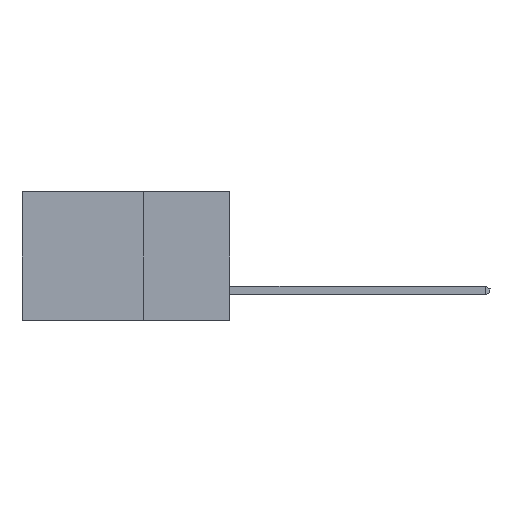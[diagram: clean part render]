
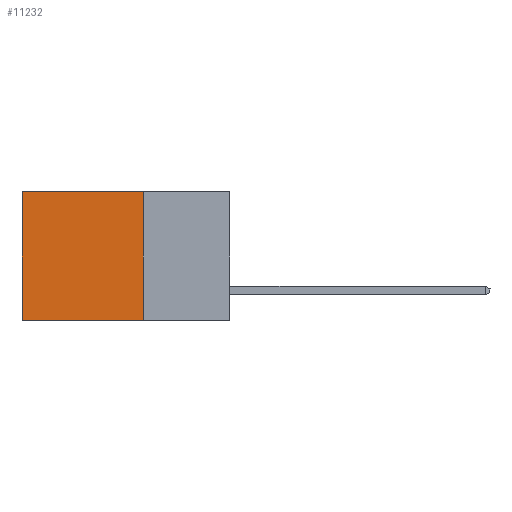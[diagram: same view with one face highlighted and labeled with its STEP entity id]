
A CAD part, left-side view. The second image highlights one B-rep face of the part: STEP entity #11232.
In plain terms, the highlighted planar face has unit normal (-1, 0, 0).
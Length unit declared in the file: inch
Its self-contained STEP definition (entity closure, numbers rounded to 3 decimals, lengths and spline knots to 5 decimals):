
#88 = LINE ( 'NONE', #11737, #9598 ) ;
#199 = DIRECTION ( 'NONE',  ( 0., 1., 0. ) ) ;
#221 = DIRECTION ( 'NONE',  ( 0., 0., -1. ) ) ;
#704 = DIRECTION ( 'NONE',  ( 0., 0., -1. ) ) ;
#1041 = LINE ( 'NONE', #12473, #8556 ) ;
#1166 = EDGE_CURVE ( 'NONE', #5690, #11440, #5392, .T. ) ;
#1561 = VECTOR ( 'NONE', #11992, 39.37008 ) ;
#1799 = ORIENTED_EDGE ( 'NONE', *, *, #5631, .F. ) ;
#2341 = CARTESIAN_POINT ( 'NONE',  ( 0.2615, 0.6, -0.37 ) ) ;
#3004 = CARTESIAN_POINT ( 'NONE',  ( 0.2615, 0.6, 0. ) ) ;
#3561 = VERTEX_POINT ( 'NONE', #3004 ) ;
#3875 = ORIENTED_EDGE ( 'NONE', *, *, #1166, .F. ) ;
#3984 = DIRECTION ( 'NONE',  ( 1., 0., 0. ) ) ;
#4280 = CARTESIAN_POINT ( 'NONE',  ( 0.2615, 0.25, -0.37 ) ) ;
#5392 = LINE ( 'NONE', #9681, #10831 ) ;
#5631 = EDGE_CURVE ( 'NONE', #10891, #5690, #88, .T. ) ;
#5690 = VERTEX_POINT ( 'NONE', #4280 ) ;
#5800 = CARTESIAN_POINT ( 'NONE',  ( 0.2615, 0.25, 0. ) ) ;
#6017 = PLANE ( 'NONE',  #13345 ) ;
#6875 = LINE ( 'NONE', #5800, #1561 ) ;
#7018 = EDGE_CURVE ( 'NONE', #10891, #3561, #6875, .T. ) ;
#7914 = EDGE_CURVE ( 'NONE', #3561, #11440, #1041, .T. ) ;
#7997 = FACE_OUTER_BOUND ( 'NONE', #12380, .T. ) ;
#8160 = ORIENTED_EDGE ( 'NONE', *, *, #7914, .T. ) ;
#8207 = DIRECTION ( 'NONE',  ( 0., 0., -1. ) ) ;
#8556 = VECTOR ( 'NONE', #8207, 39.37008 ) ;
#9427 = CARTESIAN_POINT ( 'NONE',  ( 0.2615, 0.25, 0. ) ) ;
#9598 = VECTOR ( 'NONE', #221, 39.37008 ) ;
#9681 = CARTESIAN_POINT ( 'NONE',  ( 0.2615, 0.25, -0.37 ) ) ;
#10831 = VECTOR ( 'NONE', #199, 39.37008 ) ;
#10891 = VERTEX_POINT ( 'NONE', #9427 ) ;
#10917 = ORIENTED_EDGE ( 'NONE', *, *, #7018, .T. ) ;
#11034 = CARTESIAN_POINT ( 'NONE',  ( 0.2615, 0.25, -0.37 ) ) ;
#11232 = ADVANCED_FACE ( 'NONE', ( #7997 ), #6017, .F. ) ;
#11440 = VERTEX_POINT ( 'NONE', #2341 ) ;
#11737 = CARTESIAN_POINT ( 'NONE',  ( 0.2615, 0.25, -0.37 ) ) ;
#11992 = DIRECTION ( 'NONE',  ( 0., 1., 0. ) ) ;
#12380 = EDGE_LOOP ( 'NONE', ( #8160, #3875, #1799, #10917 ) ) ;
#12473 = CARTESIAN_POINT ( 'NONE',  ( 0.2615, 0.6, -0.37 ) ) ;
#13345 = AXIS2_PLACEMENT_3D ( 'NONE', #11034, #3984, #704 ) ;
